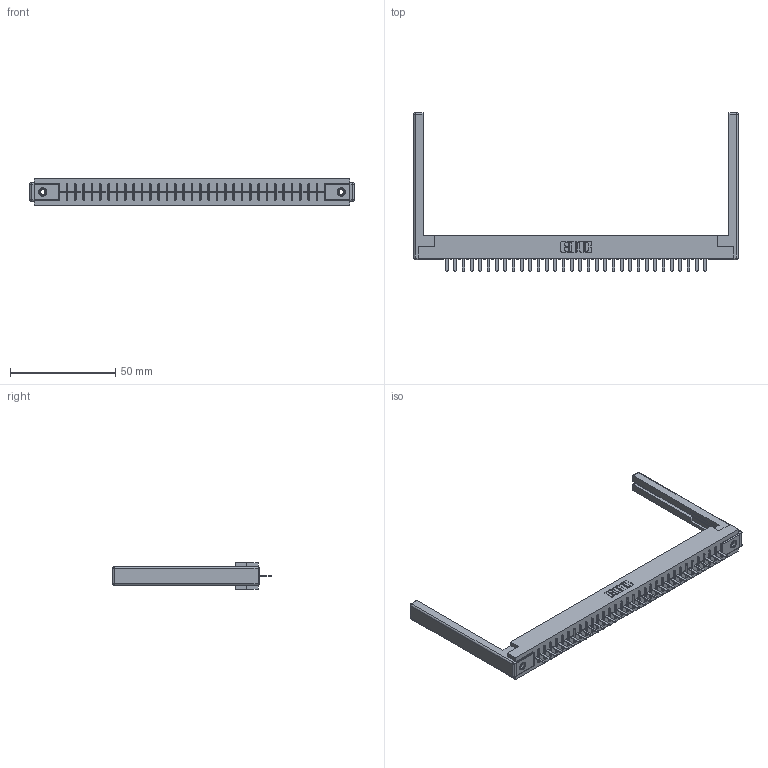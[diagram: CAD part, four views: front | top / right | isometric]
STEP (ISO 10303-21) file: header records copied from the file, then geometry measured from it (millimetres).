
FILE_DESCRIPTION (( 'STEP AP203' ), '1' );
FILE_NAME ('356-032-420-168.STEP', '2020-09-23T21:18:00', ( '' ), ( '' ), 'SwSTEP 2.0', 'SolidWorks 2020', '' );
FILE_SCHEMA (( 'CONFIG_CONTROL_DESIGN' ));
Length unit declared in the file: inch
Products named in the file (5): 306-290-001_120; 306 Part_.156 Dia; 356-032-420-168; 307-220-068; 345-250-001_345-250-001-102
Assembly tree (37 placements, depth 2):
  356-032-420-168
    306 Part_.156 Dia
    306-290-001_120  x32
    345-250-001_345-250-001-102  x2
    307-220-068  x2
Bounding box: 154.23 x 75.41 x 12.7 mm (x, y, z)
Volume: 21328.8 mm3; surface area: 21383.8 mm2
Topology: 37 solids, 37 shells, 2510 faces, 7010 edges, 4480 vertices
Faces by surface type: plane 1660, cylinder 698, sphere 136, cone 12, torus 4
Entity records: 33852 total; most frequent: CARTESIAN_POINT 5648, ORIENTED_EDGE 5590, DIRECTION 5583, EDGE_CURVE 2795, VECTOR 2177, LINE 2177, VERTEX_POINT 1768, AXIS2_PLACEMENT_3D 1703
